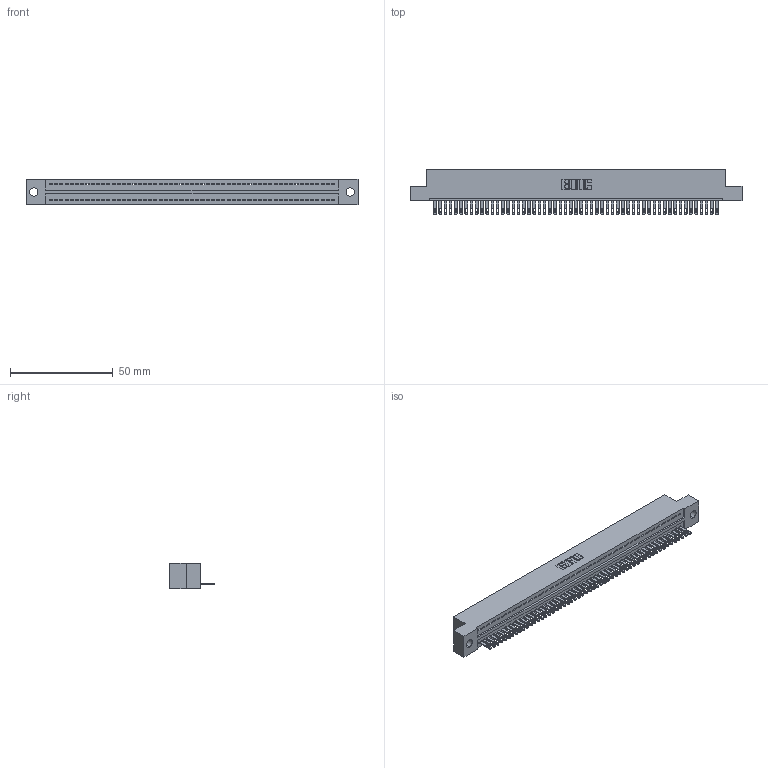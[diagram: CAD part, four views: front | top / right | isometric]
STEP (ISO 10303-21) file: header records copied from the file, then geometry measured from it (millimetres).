
FILE_DESCRIPTION (( 'STEP AP203' ), '1' );
FILE_NAME ('325-055-500-109.STEP', '2020-02-25T01:09:10', ( '' ), ( '' ), 'SwSTEP 2.0', 'SolidWorks 2016', '' );
FILE_SCHEMA (( 'CONFIG_CONTROL_DESIGN' ));
Length unit declared in the file: inch
Products named in the file (3): 325 Part_.160 TH; 325-292-001_325-293-100; 325-055-500-109
Assembly tree (56 placements, depth 2):
  325-055-500-109
    325 Part_.160 TH
    325-292-001_325-293-100  x55
Bounding box: 161.42 x 21.84 x 12.45 mm (x, y, z)
Volume: 20397.5 mm3; surface area: 22529.3 mm2
Topology: 56 solids, 56 shells, 3084 faces, 9551 edges, 6366 vertices
Faces by surface type: plane 2050, cylinder 1034
Entity records: 31875 total; most frequent: CARTESIAN_POINT 5503, ORIENTED_EDGE 5494, DIRECTION 4617, EDGE_CURVE 2747, LINE 2615, VECTOR 2615, VERTEX_POINT 1830, AXIS2_PLACEMENT_3D 1001
